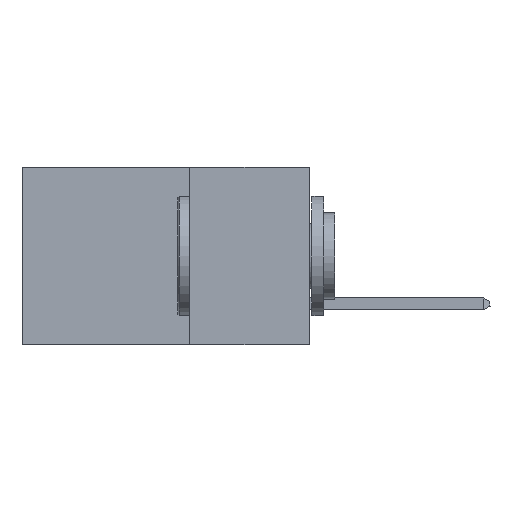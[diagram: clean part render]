
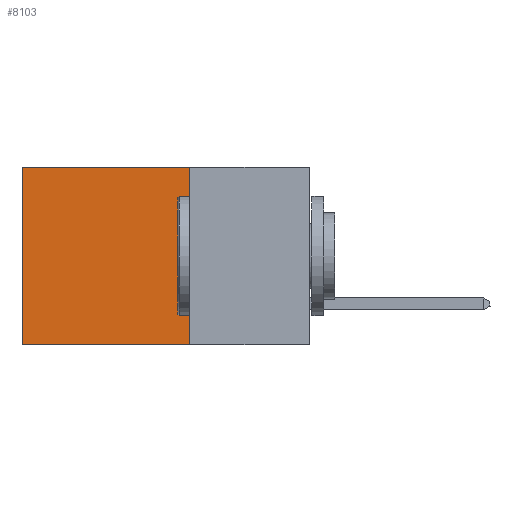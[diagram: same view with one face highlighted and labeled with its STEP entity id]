
A CAD part, left-side view. The second image highlights one B-rep face of the part: STEP entity #8103.
In plain terms, the highlighted planar face has unit normal (-1, 0, 0).
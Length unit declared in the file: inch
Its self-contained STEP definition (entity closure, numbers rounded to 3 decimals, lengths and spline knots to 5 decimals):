
#23 = CARTESIAN_POINT ( 'NONE',  ( 0.2875, 0.6, 0. ) ) ;
#2232 = CARTESIAN_POINT ( 'NONE',  ( 0.2875, 0.6, -0.37 ) ) ;
#3642 = DIRECTION ( 'NONE',  ( 0., 0., -1. ) ) ;
#4265 = VECTOR ( 'NONE', #25393, 39.37008 ) ;
#4900 = LINE ( 'NONE', #7122, #30334 ) ;
#7068 = EDGE_CURVE ( 'NONE', #36328, #44428, #17504, .T. ) ;
#7122 = CARTESIAN_POINT ( 'NONE',  ( 0.2875, 0.25, 0. ) ) ;
#7182 = DIRECTION ( 'NONE',  ( 0., 0., -1. ) ) ;
#8103 = ADVANCED_FACE ( 'NONE', ( #26859 ), #41197, .F. ) ;
#13779 = DIRECTION ( 'NONE',  ( 0., 1., 0. ) ) ;
#17504 = LINE ( 'NONE', #23, #47688 ) ;
#17667 = ORIENTED_EDGE ( 'NONE', *, *, #37618, .T. ) ;
#18832 = CARTESIAN_POINT ( 'NONE',  ( 0.2875, 0.25, 0. ) ) ;
#19305 = VERTEX_POINT ( 'NONE', #33281 ) ;
#21018 = EDGE_CURVE ( 'NONE', #44701, #19305, #4900, .T. ) ;
#22532 = CARTESIAN_POINT ( 'NONE',  ( 0.2875, 0.25, 0. ) ) ;
#23195 = LINE ( 'NONE', #48045, #4265 ) ;
#23614 = LINE ( 'NONE', #28989, #40137 ) ;
#24652 = EDGE_CURVE ( 'NONE', #19305, #44428, #23614, .T. ) ;
#25393 = DIRECTION ( 'NONE',  ( 0., 1., 0. ) ) ;
#25966 = EDGE_LOOP ( 'NONE', ( #38611, #42745, #29321, #17667 ) ) ;
#26859 = FACE_OUTER_BOUND ( 'NONE', #25966, .T. ) ;
#28989 = CARTESIAN_POINT ( 'NONE',  ( 0.2875, 0.25, -0.37 ) ) ;
#29321 = ORIENTED_EDGE ( 'NONE', *, *, #21018, .F. ) ;
#30334 = VECTOR ( 'NONE', #3642, 39.37008 ) ;
#33281 = CARTESIAN_POINT ( 'NONE',  ( 0.2875, 0.25, -0.37 ) ) ;
#36328 = VERTEX_POINT ( 'NONE', #46905 ) ;
#37538 = DIRECTION ( 'NONE',  ( 1., 0., 0. ) ) ;
#37618 = EDGE_CURVE ( 'NONE', #44701, #36328, #23195, .T. ) ;
#38611 = ORIENTED_EDGE ( 'NONE', *, *, #7068, .T. ) ;
#40137 = VECTOR ( 'NONE', #13779, 39.37008 ) ;
#41197 = PLANE ( 'NONE',  #44221 ) ;
#42745 = ORIENTED_EDGE ( 'NONE', *, *, #24652, .F. ) ;
#44221 = AXIS2_PLACEMENT_3D ( 'NONE', #22532, #37538, #7182 ) ;
#44428 = VERTEX_POINT ( 'NONE', #2232 ) ;
#44701 = VERTEX_POINT ( 'NONE', #18832 ) ;
#45605 = DIRECTION ( 'NONE',  ( 0., 0., -1. ) ) ;
#46905 = CARTESIAN_POINT ( 'NONE',  ( 0.2875, 0.6, 0. ) ) ;
#47688 = VECTOR ( 'NONE', #45605, 39.37008 ) ;
#48045 = CARTESIAN_POINT ( 'NONE',  ( 0.2875, 0.25, 0. ) ) ;
